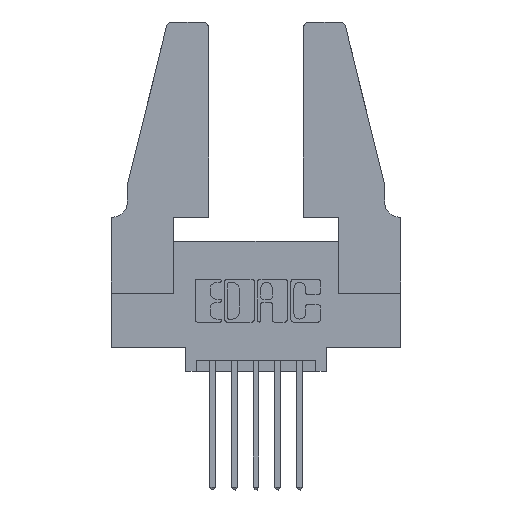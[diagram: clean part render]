
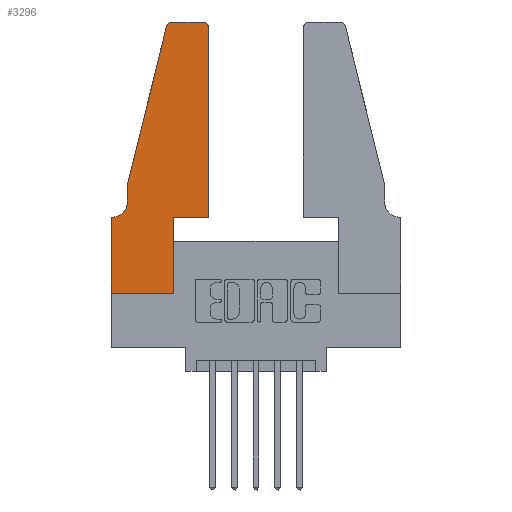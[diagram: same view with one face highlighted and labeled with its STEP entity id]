
A CAD part, top view. The second image highlights one B-rep face of the part: STEP entity #3296.
In plain terms, the highlighted planar face has unit normal (0, 0, 1).
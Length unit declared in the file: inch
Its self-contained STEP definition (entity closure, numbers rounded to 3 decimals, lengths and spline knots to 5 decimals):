
#9 = VECTOR ( 'NONE', #2755, 39.37008 ) ;
#57 = VERTEX_POINT ( 'NONE', #5098 ) ;
#68 = CARTESIAN_POINT ( 'NONE',  ( 0.25487, 1.22718, 0.37 ) ) ;
#255 = EDGE_CURVE ( 'NONE', #11080, #57, #900, .T. ) ;
#270 = ORIENTED_EDGE ( 'NONE', *, *, #9726, .T. ) ;
#347 = VERTEX_POINT ( 'NONE', #1901 ) ;
#408 = CARTESIAN_POINT ( 'NONE',  ( 0.0755, 0.35, 0.37 ) ) ;
#558 = ORIENTED_EDGE ( 'NONE', *, *, #6767, .T. ) ;
#613 = PLANE ( 'NONE',  #1168 ) ;
#728 = VERTEX_POINT ( 'NONE', #1704 ) ;
#806 = DIRECTION ( 'NONE',  ( 1., 0., 0. ) ) ;
#898 = EDGE_CURVE ( 'NONE', #347, #11080, #10463, .T. ) ;
#900 = LINE ( 'NONE', #10031, #7342 ) ;
#1066 = LINE ( 'NONE', #7626, #7743 ) ;
#1104 = EDGE_CURVE ( 'NONE', #57, #6383, #4052, .T. ) ;
#1168 = AXIS2_PLACEMENT_3D ( 'NONE', #5951, #3335, #9356 ) ;
#1280 = EDGE_CURVE ( 'NONE', #10754, #347, #7318, .T. ) ;
#1330 = DIRECTION ( 'NONE',  ( -1., 0., 0. ) ) ;
#1426 = LINE ( 'NONE', #4393, #6096 ) ;
#1554 = VERTEX_POINT ( 'NONE', #68 ) ;
#1704 = CARTESIAN_POINT ( 'NONE',  ( 0.284, 1.25, 0.37 ) ) ;
#1720 = CARTESIAN_POINT ( 'NONE',  ( 0.4505, 0.35, 0.37 ) ) ;
#1748 = AXIS2_PLACEMENT_3D ( 'NONE', #11127, #6093, #806 ) ;
#1901 = CARTESIAN_POINT ( 'NONE',  ( 0.2865, 0., 0.37 ) ) ;
#1933 = EDGE_CURVE ( 'NONE', #728, #1554, #3344, .T. ) ;
#2140 = DIRECTION ( 'NONE',  ( 0., 1., 0. ) ) ;
#2206 = CARTESIAN_POINT ( 'NONE',  ( 0., 0., 0.37 ) ) ;
#2264 = CARTESIAN_POINT ( 'NONE',  ( 0.0055, 0.35, 0.37 ) ) ;
#2445 = ORIENTED_EDGE ( 'NONE', *, *, #1280, .T. ) ;
#2552 = VERTEX_POINT ( 'NONE', #7999 ) ;
#2733 = DIRECTION ( 'NONE',  ( 1., 0., 0. ) ) ;
#2755 = DIRECTION ( 'NONE',  ( 0., -1., 0. ) ) ;
#2807 = EDGE_CURVE ( 'NONE', #8945, #728, #1426, .T. ) ;
#2811 = ORIENTED_EDGE ( 'NONE', *, *, #10353, .T. ) ;
#2840 = VERTEX_POINT ( 'NONE', #3572 ) ;
#3072 = DIRECTION ( 'NONE',  ( 0., 0., -1. ) ) ;
#3094 = EDGE_CURVE ( 'NONE', #2840, #7989, #5952, .T. ) ;
#3270 = AXIS2_PLACEMENT_3D ( 'NONE', #8925, #8920, #7633 ) ;
#3296 = ADVANCED_FACE ( 'NONE', ( #10563 ), #613, .T. ) ;
#3332 = CARTESIAN_POINT ( 'NONE',  ( 0., 0.35, 0.37 ) ) ;
#3335 = DIRECTION ( 'NONE',  ( 0., 0., 1. ) ) ;
#3344 = CIRCLE ( 'NONE', #3270, 0.03 ) ;
#3572 = CARTESIAN_POINT ( 'NONE',  ( 0.0755, 0.42, 0.37 ) ) ;
#3646 = VECTOR ( 'NONE', #7479, 39.37008 ) ;
#3661 = ORIENTED_EDGE ( 'NONE', *, *, #1933, .T. ) ;
#4052 = LINE ( 'NONE', #1720, #6387 ) ;
#4393 = CARTESIAN_POINT ( 'NONE',  ( 0.2605, 1.25, 0.37 ) ) ;
#4583 = ORIENTED_EDGE ( 'NONE', *, *, #6462, .T. ) ;
#4751 = VECTOR ( 'NONE', #5448, 39.37008 ) ;
#4922 = AXIS2_PLACEMENT_3D ( 'NONE', #8257, #3072, #9100 ) ;
#4977 = VECTOR ( 'NONE', #5330, 39.37008 ) ;
#5098 = CARTESIAN_POINT ( 'NONE',  ( 0.4505, 0.35, 0.37 ) ) ;
#5183 = ORIENTED_EDGE ( 'NONE', *, *, #3094, .T. ) ;
#5230 = ORIENTED_EDGE ( 'NONE', *, *, #10484, .T. ) ;
#5330 = DIRECTION ( 'NONE',  ( 0., -1., 0. ) ) ;
#5346 = CARTESIAN_POINT ( 'NONE',  ( 0.2865, 0.35, 0.37 ) ) ;
#5448 = DIRECTION ( 'NONE',  ( 1., 0., 0. ) ) ;
#5882 = ORIENTED_EDGE ( 'NONE', *, *, #2807, .T. ) ;
#5951 = CARTESIAN_POINT ( 'NONE',  ( 0., 0.35, 0.37 ) ) ;
#5952 = CIRCLE ( 'NONE', #4922, 0.07 ) ;
#6093 = DIRECTION ( 'NONE',  ( 0., 0., 1. ) ) ;
#6096 = VECTOR ( 'NONE', #11186, 39.37008 ) ;
#6257 = VERTEX_POINT ( 'NONE', #3332 ) ;
#6383 = VERTEX_POINT ( 'NONE', #11169 ) ;
#6387 = VECTOR ( 'NONE', #2140, 39.37008 ) ;
#6462 = EDGE_CURVE ( 'NONE', #6257, #10754, #10287, .T. ) ;
#6767 = EDGE_CURVE ( 'NONE', #7989, #6257, #6864, .T. ) ;
#6864 = LINE ( 'NONE', #408, #11066 ) ;
#7067 = LINE ( 'NONE', #8800, #9 ) ;
#7318 = LINE ( 'NONE', #8023, #4751 ) ;
#7342 = VECTOR ( 'NONE', #2733, 39.37008 ) ;
#7443 = CARTESIAN_POINT ( 'NONE',  ( 0.2865, 0.35, 0.37 ) ) ;
#7479 = DIRECTION ( 'NONE',  ( 0., 1., 0. ) ) ;
#7626 = CARTESIAN_POINT ( 'NONE',  ( 0.0755, 0.5, 0.37 ) ) ;
#7633 = DIRECTION ( 'NONE',  ( 1., 0., 0. ) ) ;
#7743 = VECTOR ( 'NONE', #8469, 39.37008 ) ;
#7989 = VERTEX_POINT ( 'NONE', #2264 ) ;
#7999 = CARTESIAN_POINT ( 'NONE',  ( 0.0755, 0.5, 0.37 ) ) ;
#8023 = CARTESIAN_POINT ( 'NONE',  ( 0., 0., 0.37 ) ) ;
#8257 = CARTESIAN_POINT ( 'NONE',  ( 0.0055, 0.42, 0.37 ) ) ;
#8424 = ORIENTED_EDGE ( 'NONE', *, *, #1104, .T. ) ;
#8469 = DIRECTION ( 'NONE',  ( -0.239, -0.971, 0. ) ) ;
#8691 = EDGE_LOOP ( 'NONE', ( #5882, #3661, #270, #5230, #5183, #558, #4583, #2445, #10022, #9807, #8424, #2811 ) ) ;
#8800 = CARTESIAN_POINT ( 'NONE',  ( 0.0755, 0.5, 0.37 ) ) ;
#8920 = DIRECTION ( 'NONE',  ( 0., 0., 1. ) ) ;
#8925 = CARTESIAN_POINT ( 'NONE',  ( 0.284, 1.22, 0.37 ) ) ;
#8945 = VERTEX_POINT ( 'NONE', #10722 ) ;
#9100 = DIRECTION ( 'NONE',  ( -1., 0., 0. ) ) ;
#9356 = DIRECTION ( 'NONE',  ( 1., 0., 0. ) ) ;
#9603 = CARTESIAN_POINT ( 'NONE',  ( 0., 0., 0.37 ) ) ;
#9726 = EDGE_CURVE ( 'NONE', #1554, #2552, #1066, .T. ) ;
#9807 = ORIENTED_EDGE ( 'NONE', *, *, #255, .T. ) ;
#10022 = ORIENTED_EDGE ( 'NONE', *, *, #898, .T. ) ;
#10031 = CARTESIAN_POINT ( 'NONE',  ( 0.4505, 0.35, 0.37 ) ) ;
#10287 = LINE ( 'NONE', #9603, #4977 ) ;
#10353 = EDGE_CURVE ( 'NONE', #6383, #8945, #10617, .T. ) ;
#10463 = LINE ( 'NONE', #7443, #3646 ) ;
#10484 = EDGE_CURVE ( 'NONE', #2552, #2840, #7067, .T. ) ;
#10563 = FACE_OUTER_BOUND ( 'NONE', #8691, .T. ) ;
#10617 = CIRCLE ( 'NONE', #1748, 0.03 ) ;
#10722 = CARTESIAN_POINT ( 'NONE',  ( 0.4205, 1.25, 0.37 ) ) ;
#10754 = VERTEX_POINT ( 'NONE', #2206 ) ;
#11066 = VECTOR ( 'NONE', #1330, 39.37008 ) ;
#11080 = VERTEX_POINT ( 'NONE', #5346 ) ;
#11127 = CARTESIAN_POINT ( 'NONE',  ( 0.4205, 1.22, 0.37 ) ) ;
#11169 = CARTESIAN_POINT ( 'NONE',  ( 0.4505, 1.22, 0.37 ) ) ;
#11186 = DIRECTION ( 'NONE',  ( -1., 0., 0. ) ) ;
